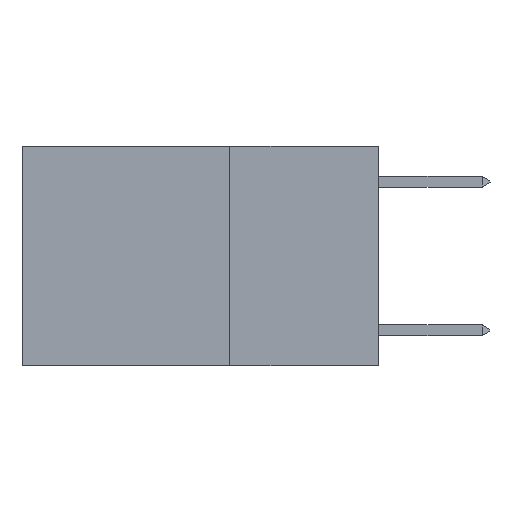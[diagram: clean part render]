
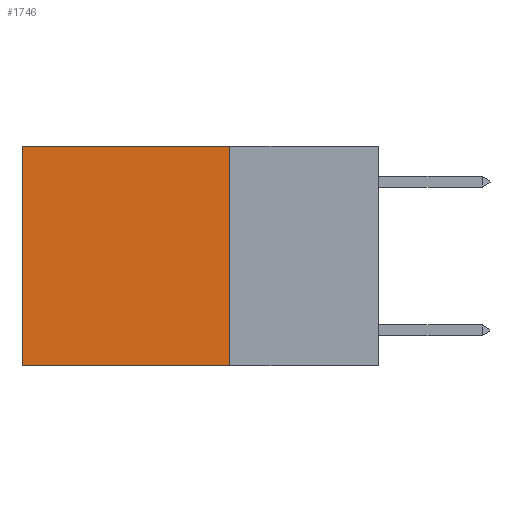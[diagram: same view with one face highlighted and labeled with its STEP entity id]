
A CAD part, left-side view. The second image highlights one B-rep face of the part: STEP entity #1746.
In plain terms, the highlighted planar face has unit normal (-1, 0, 0).
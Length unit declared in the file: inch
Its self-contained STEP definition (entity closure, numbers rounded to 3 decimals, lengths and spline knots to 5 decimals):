
#1070 = CARTESIAN_POINT ( 'NONE',  ( 0.2625, 0.25, 0. ) ) ;
#1373 = CARTESIAN_POINT ( 'NONE',  ( 0.2625, 0.6, -0.37 ) ) ;
#1421 = VERTEX_POINT ( 'NONE', #9839 ) ;
#1444 = DIRECTION ( 'NONE',  ( 0., 1., 0. ) ) ;
#1612 = ORIENTED_EDGE ( 'NONE', *, *, #13406, .T. ) ;
#1746 = ADVANCED_FACE ( 'NONE', ( #11063 ), #6047, .F. ) ;
#1856 = LINE ( 'NONE', #8073, #6756 ) ;
#1890 = ORIENTED_EDGE ( 'NONE', *, *, #12194, .F. ) ;
#2245 = ORIENTED_EDGE ( 'NONE', *, *, #13530, .F. ) ;
#2416 = ORIENTED_EDGE ( 'NONE', *, *, #13148, .T. ) ;
#3279 = VECTOR ( 'NONE', #5133, 39.37008 ) ;
#3404 = AXIS2_PLACEMENT_3D ( 'NONE', #8702, #5970, #5762 ) ;
#3414 = VERTEX_POINT ( 'NONE', #1373 ) ;
#3823 = VECTOR ( 'NONE', #12741, 39.37008 ) ;
#4101 = CARTESIAN_POINT ( 'NONE',  ( 0.2625, 0.25, 0. ) ) ;
#4174 = LINE ( 'NONE', #11673, #3823 ) ;
#5133 = DIRECTION ( 'NONE',  ( 0., 0., -1. ) ) ;
#5762 = DIRECTION ( 'NONE',  ( 0., 0., -1. ) ) ;
#5970 = DIRECTION ( 'NONE',  ( 1., 0., 0. ) ) ;
#6047 = PLANE ( 'NONE',  #3404 ) ;
#6620 = CARTESIAN_POINT ( 'NONE',  ( 0.2625, 0.25, 0. ) ) ;
#6756 = VECTOR ( 'NONE', #10089, 39.37008 ) ;
#8073 = CARTESIAN_POINT ( 'NONE',  ( 0.2625, 0.6, 0. ) ) ;
#8444 = VERTEX_POINT ( 'NONE', #11698 ) ;
#8702 = CARTESIAN_POINT ( 'NONE',  ( 0.2625, 0.25, 0. ) ) ;
#9211 = LINE ( 'NONE', #4101, #3279 ) ;
#9839 = CARTESIAN_POINT ( 'NONE',  ( 0.2625, 0.6, 0. ) ) ;
#10038 = VECTOR ( 'NONE', #1444, 39.37008 ) ;
#10089 = DIRECTION ( 'NONE',  ( 0., 0., -1. ) ) ;
#11052 = EDGE_LOOP ( 'NONE', ( #1612, #1890, #2245, #2416 ) ) ;
#11063 = FACE_OUTER_BOUND ( 'NONE', #11052, .T. ) ;
#11673 = CARTESIAN_POINT ( 'NONE',  ( 0.2625, 0.25, -0.37 ) ) ;
#11698 = CARTESIAN_POINT ( 'NONE',  ( 0.2625, 0.25, -0.37 ) ) ;
#12194 = EDGE_CURVE ( 'NONE', #8444, #3414, #4174, .T. ) ;
#12741 = DIRECTION ( 'NONE',  ( 0., 1., 0. ) ) ;
#12796 = LINE ( 'NONE', #6620, #10038 ) ;
#12846 = VERTEX_POINT ( 'NONE', #1070 ) ;
#13148 = EDGE_CURVE ( 'NONE', #12846, #1421, #12796, .T. ) ;
#13406 = EDGE_CURVE ( 'NONE', #1421, #3414, #1856, .T. ) ;
#13530 = EDGE_CURVE ( 'NONE', #12846, #8444, #9211, .T. ) ;
